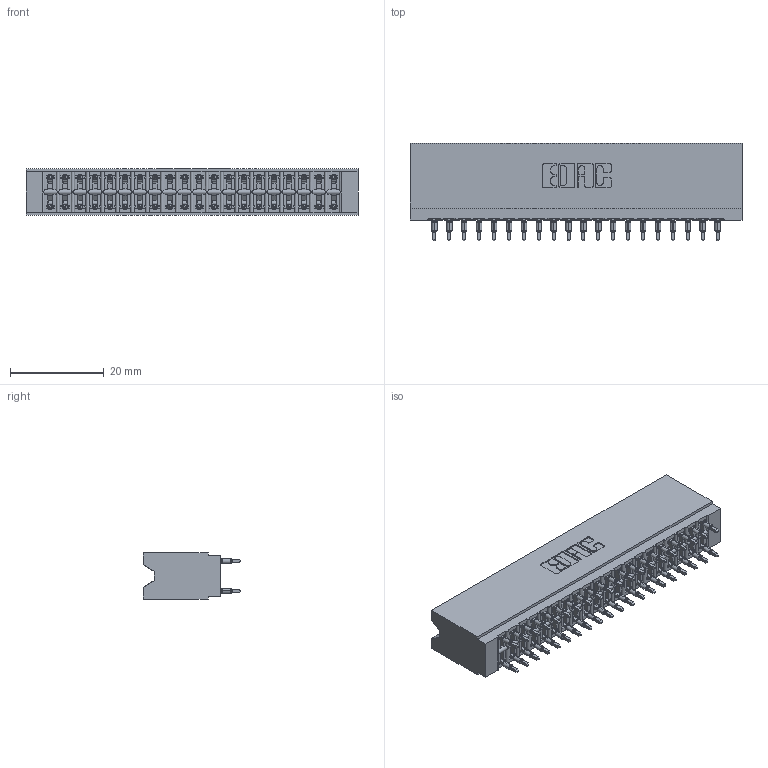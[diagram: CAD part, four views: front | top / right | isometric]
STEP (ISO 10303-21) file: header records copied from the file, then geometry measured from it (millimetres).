
FILE_DESCRIPTION (( 'STEP AP203' ), '1' );
FILE_NAME ('746-040-560-206.STEP', '2020-09-16T18:47:51', ( '' ), ( '' ), 'SwSTEP 2.0', 'SolidWorks 2020', '' );
FILE_SCHEMA (( 'CONFIG_CONTROL_DESIGN' ));
Length unit declared in the file: inch
Products named in the file (3): 746-292-001_560; 746-040-560-206; 746 Part_.515 Slot Depth - 06
Assembly tree (41 placements, depth 2):
  746-040-560-206
    746 Part_.515 Slot Depth - 06
    746-292-001_560  x40
Bounding box: 70.74 x 20.82 x 9.91 mm (x, y, z)
Volume: 7854 mm3; surface area: 12940.3 mm2
Topology: 41 solids, 41 shells, 3878 faces, 10785 edges, 6915 vertices
Faces by surface type: plane 1936, cylinder 902, bspline 800, torus 240
Entity records: 34182 total; most frequent: CARTESIAN_POINT 6982, ORIENTED_EDGE 5814, DIRECTION 4899, EDGE_CURVE 2907, LINE 2515, VECTOR 2515, VERTEX_POINT 1923, AXIS2_PLACEMENT_3D 1192
